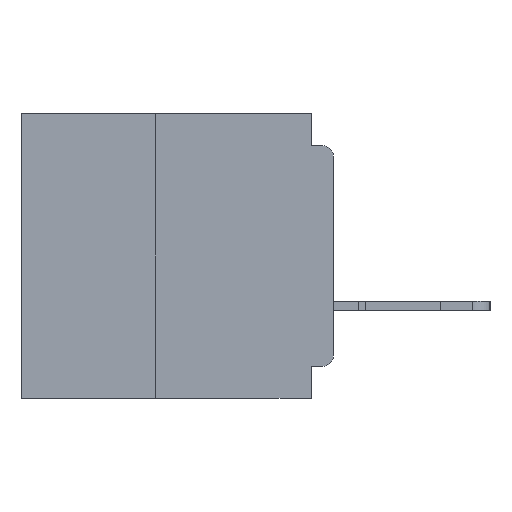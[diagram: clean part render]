
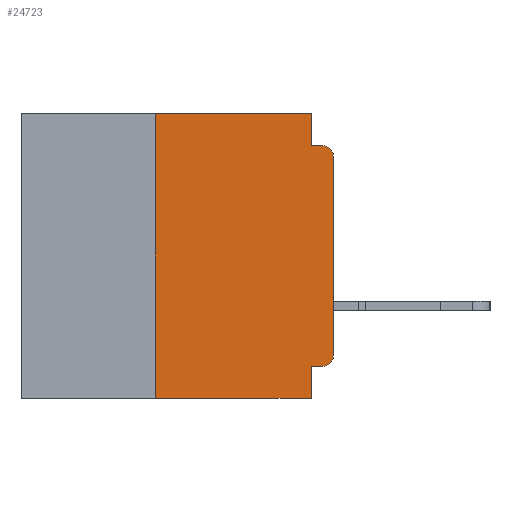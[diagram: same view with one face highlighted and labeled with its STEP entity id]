
A CAD part, left-side view. The second image highlights one B-rep face of the part: STEP entity #24723.
In plain terms, the highlighted planar face has unit normal (-1, 0, 0).
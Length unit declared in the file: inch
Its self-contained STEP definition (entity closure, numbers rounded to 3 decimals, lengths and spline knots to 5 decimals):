
#564 = ORIENTED_EDGE ( 'NONE', *, *, #53142, .T. ) ;
#2126 = EDGE_CURVE ( 'NONE', #12410, #15601, #44708, .T. ) ;
#2852 = CARTESIAN_POINT ( 'NONE',  ( 0., 0.015, -0.34 ) ) ;
#2933 = AXIS2_PLACEMENT_3D ( 'NONE', #2852, #38201, #7981 ) ;
#3618 = VECTOR ( 'NONE', #22258, 39.37008 ) ;
#5795 = LINE ( 'NONE', #57150, #57743 ) ;
#7213 = CARTESIAN_POINT ( 'NONE',  ( 0., 0.015, -0.045 ) ) ;
#7981 = DIRECTION ( 'NONE',  ( 0., 0., -1. ) ) ;
#8328 = VECTOR ( 'NONE', #57706, 39.37008 ) ;
#10849 = PLANE ( 'NONE',  #56452 ) ;
#11197 = FACE_OUTER_BOUND ( 'NONE', #21038, .T. ) ;
#11561 = VERTEX_POINT ( 'NONE', #26633 ) ;
#11778 = ORIENTED_EDGE ( 'NONE', *, *, #2126, .F. ) ;
#12410 = VERTEX_POINT ( 'NONE', #42305 ) ;
#14725 = DIRECTION ( 'NONE',  ( 0., 0., -1. ) ) ;
#15601 = VERTEX_POINT ( 'NONE', #7213 ) ;
#17098 = CARTESIAN_POINT ( 'NONE',  ( 0., 0.25, -0.4 ) ) ;
#17152 = DIRECTION ( 'NONE',  ( 0., 0., -1. ) ) ;
#17163 = CARTESIAN_POINT ( 'NONE',  ( 0., 0.437, 0. ) ) ;
#17348 = CARTESIAN_POINT ( 'NONE',  ( 0., 0.031, -0.355 ) ) ;
#17708 = LINE ( 'NONE', #61018, #29574 ) ;
#17946 = VERTEX_POINT ( 'NONE', #17348 ) ;
#17965 = EDGE_CURVE ( 'NONE', #39570, #58102, #18439, .T. ) ;
#18439 = LINE ( 'NONE', #32350, #43602 ) ;
#18951 = CARTESIAN_POINT ( 'NONE',  ( 0., 0., -0.045 ) ) ;
#20798 = ORIENTED_EDGE ( 'NONE', *, *, #17965, .T. ) ;
#21038 = EDGE_LOOP ( 'NONE', ( #61691, #34255, #11778, #46302, #30260, #29509, #20798, #37750, #49530, #564 ) ) ;
#21119 = DIRECTION ( 'NONE',  ( 0., 0., 1. ) ) ;
#21243 = CARTESIAN_POINT ( 'NONE',  ( 0., 0.437, 0. ) ) ;
#22090 = CARTESIAN_POINT ( 'NONE',  ( 0., 0.015, -0.06 ) ) ;
#22258 = DIRECTION ( 'NONE',  ( 0., -1., 0. ) ) ;
#22978 = EDGE_CURVE ( 'NONE', #61771, #15601, #63973, .T. ) ;
#23303 = VERTEX_POINT ( 'NONE', #59765 ) ;
#23495 = CIRCLE ( 'NONE', #2933, 0.015 ) ;
#24723 = ADVANCED_FACE ( 'NONE', ( #11197 ), #10849, .F. ) ;
#26318 = DIRECTION ( 'NONE',  ( 1., 0., 0. ) ) ;
#26528 = LINE ( 'NONE', #52702, #8328 ) ;
#26633 = CARTESIAN_POINT ( 'NONE',  ( 0., 0.015, -0.355 ) ) ;
#26686 = CARTESIAN_POINT ( 'NONE',  ( 0., 0.031, -0.4 ) ) ;
#27158 = DIRECTION ( 'NONE',  ( 0., 0., -1. ) ) ;
#29509 = ORIENTED_EDGE ( 'NONE', *, *, #61502, .F. ) ;
#29574 = VECTOR ( 'NONE', #21119, 39.37008 ) ;
#29957 = DIRECTION ( 'NONE',  ( 0., 1., 0. ) ) ;
#30260 = ORIENTED_EDGE ( 'NONE', *, *, #32375, .F. ) ;
#30483 = EDGE_CURVE ( 'NONE', #17946, #58102, #39475, .T. ) ;
#31405 = VECTOR ( 'NONE', #54120, 39.37008 ) ;
#32350 = CARTESIAN_POINT ( 'NONE',  ( 0., 0.437, -0.4 ) ) ;
#32375 = EDGE_CURVE ( 'NONE', #64836, #48906, #43863, .T. ) ;
#32420 = VECTOR ( 'NONE', #29957, 39.37008 ) ;
#32566 = DIRECTION ( 'NONE',  ( 0., -1., 0. ) ) ;
#34255 = ORIENTED_EDGE ( 'NONE', *, *, #22978, .T. ) ;
#36314 = VECTOR ( 'NONE', #14725, 39.37008 ) ;
#37593 = CARTESIAN_POINT ( 'NONE',  ( 0., 0.031, 0. ) ) ;
#37750 = ORIENTED_EDGE ( 'NONE', *, *, #30483, .F. ) ;
#38201 = DIRECTION ( 'NONE',  ( -1., 0., 0. ) ) ;
#39475 = LINE ( 'NONE', #49743, #36314 ) ;
#39570 = VERTEX_POINT ( 'NONE', #17098 ) ;
#42305 = CARTESIAN_POINT ( 'NONE',  ( 0., 0.031, -0.045 ) ) ;
#42506 = AXIS2_PLACEMENT_3D ( 'NONE', #22090, #57214, #27158 ) ;
#42608 = LINE ( 'NONE', #59922, #32420 ) ;
#43105 = CARTESIAN_POINT ( 'NONE',  ( 0., 0.25, 0. ) ) ;
#43255 = CARTESIAN_POINT ( 'NONE',  ( 0., 0., -0.06 ) ) ;
#43602 = VECTOR ( 'NONE', #32566, 39.37008 ) ;
#43863 = LINE ( 'NONE', #17163, #3618 ) ;
#44708 = LINE ( 'NONE', #18951, #31405 ) ;
#46302 = ORIENTED_EDGE ( 'NONE', *, *, #55826, .F. ) ;
#48906 = VERTEX_POINT ( 'NONE', #37593 ) ;
#49530 = ORIENTED_EDGE ( 'NONE', *, *, #64988, .F. ) ;
#49743 = CARTESIAN_POINT ( 'NONE',  ( 0., 0.031, -0.4 ) ) ;
#52702 = CARTESIAN_POINT ( 'NONE',  ( 0., 0., 0. ) ) ;
#53142 = EDGE_CURVE ( 'NONE', #11561, #23303, #23495, .T. ) ;
#54120 = DIRECTION ( 'NONE',  ( 0., -1., 0. ) ) ;
#54707 = EDGE_CURVE ( 'NONE', #23303, #61771, #26528, .T. ) ;
#55826 = EDGE_CURVE ( 'NONE', #48906, #12410, #5795, .T. ) ;
#56452 = AXIS2_PLACEMENT_3D ( 'NONE', #21243, #26318, #61359 ) ;
#57150 = CARTESIAN_POINT ( 'NONE',  ( 0., 0.031, 0. ) ) ;
#57214 = DIRECTION ( 'NONE',  ( -1., 0., 0. ) ) ;
#57706 = DIRECTION ( 'NONE',  ( 0., 0., 1. ) ) ;
#57743 = VECTOR ( 'NONE', #17152, 39.37008 ) ;
#58102 = VERTEX_POINT ( 'NONE', #26686 ) ;
#59765 = CARTESIAN_POINT ( 'NONE',  ( 0., 0., -0.34 ) ) ;
#59922 = CARTESIAN_POINT ( 'NONE',  ( 0., 0., -0.355 ) ) ;
#61018 = CARTESIAN_POINT ( 'NONE',  ( 0., 0.25, -0.4 ) ) ;
#61359 = DIRECTION ( 'NONE',  ( 0., 0., -1. ) ) ;
#61502 = EDGE_CURVE ( 'NONE', #39570, #64836, #17708, .T. ) ;
#61691 = ORIENTED_EDGE ( 'NONE', *, *, #54707, .T. ) ;
#61771 = VERTEX_POINT ( 'NONE', #43255 ) ;
#63973 = CIRCLE ( 'NONE', #42506, 0.015 ) ;
#64836 = VERTEX_POINT ( 'NONE', #43105 ) ;
#64988 = EDGE_CURVE ( 'NONE', #11561, #17946, #42608, .T. ) ;
